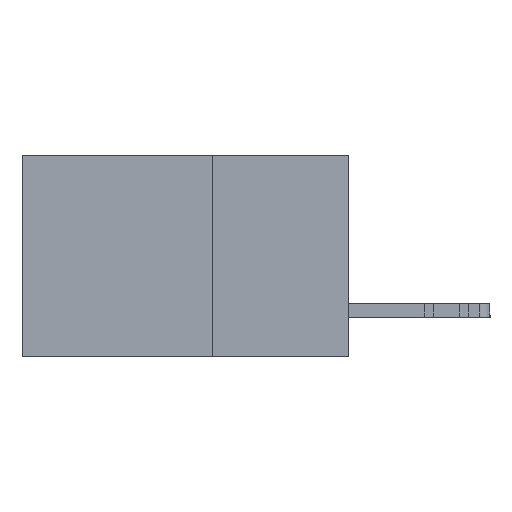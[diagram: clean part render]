
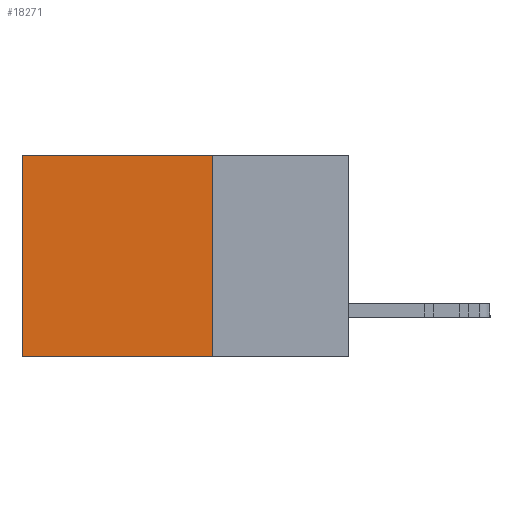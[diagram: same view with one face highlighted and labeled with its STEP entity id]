
A CAD part, left-side view. The second image highlights one B-rep face of the part: STEP entity #18271.
In plain terms, the highlighted planar face has unit normal (-1, 0, 0).
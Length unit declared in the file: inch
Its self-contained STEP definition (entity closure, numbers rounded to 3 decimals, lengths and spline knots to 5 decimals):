
#656 = LINE ( 'NONE', #15399, #14418 ) ;
#1472 = CARTESIAN_POINT ( 'NONE',  ( 0.298, 0.6, 0. ) ) ;
#2186 = EDGE_CURVE ( 'NONE', #17357, #15263, #656, .T. ) ;
#2240 = CARTESIAN_POINT ( 'NONE',  ( 0.298, 0.6, -0.37 ) ) ;
#2819 = DIRECTION ( 'NONE',  ( 1., 0., 0. ) ) ;
#4165 = DIRECTION ( 'NONE',  ( 0., 1., 0. ) ) ;
#5408 = PLANE ( 'NONE',  #13790 ) ;
#6803 = CARTESIAN_POINT ( 'NONE',  ( 0.298, 0.25, -0.37 ) ) ;
#9617 = CARTESIAN_POINT ( 'NONE',  ( 0.298, 0.25, 0. ) ) ;
#9761 = DIRECTION ( 'NONE',  ( 0., 1., 0. ) ) ;
#10037 = LINE ( 'NONE', #1472, #17065 ) ;
#10196 = VERTEX_POINT ( 'NONE', #2240 ) ;
#12437 = CARTESIAN_POINT ( 'NONE',  ( 0.298, 0.6, 0. ) ) ;
#13053 = VERTEX_POINT ( 'NONE', #6803 ) ;
#13790 = AXIS2_PLACEMENT_3D ( 'NONE', #18879, #2819, #28018 ) ;
#14145 = ORIENTED_EDGE ( 'NONE', *, *, #22791, .T. ) ;
#14226 = LINE ( 'NONE', #23444, #23072 ) ;
#14418 = VECTOR ( 'NONE', #4165, 39.37008 ) ;
#15263 = VERTEX_POINT ( 'NONE', #12437 ) ;
#15399 = CARTESIAN_POINT ( 'NONE',  ( 0.298, 0.25, 0. ) ) ;
#15647 = FACE_OUTER_BOUND ( 'NONE', #26648, .T. ) ;
#17065 = VECTOR ( 'NONE', #19205, 39.37008 ) ;
#17357 = VERTEX_POINT ( 'NONE', #9617 ) ;
#17630 = DIRECTION ( 'NONE',  ( 0., 0., -1. ) ) ;
#18271 = ADVANCED_FACE ( 'NONE', ( #15647 ), #5408, .F. ) ;
#18315 = EDGE_CURVE ( 'NONE', #13053, #10196, #14226, .T. ) ;
#18879 = CARTESIAN_POINT ( 'NONE',  ( 0.298, 0.25, 0. ) ) ;
#19205 = DIRECTION ( 'NONE',  ( 0., 0., -1. ) ) ;
#19442 = LINE ( 'NONE', #26662, #22303 ) ;
#22303 = VECTOR ( 'NONE', #17630, 39.37008 ) ;
#22791 = EDGE_CURVE ( 'NONE', #15263, #10196, #10037, .T. ) ;
#23072 = VECTOR ( 'NONE', #9761, 39.37008 ) ;
#23226 = ORIENTED_EDGE ( 'NONE', *, *, #18315, .F. ) ;
#23444 = CARTESIAN_POINT ( 'NONE',  ( 0.298, 0.25, -0.37 ) ) ;
#24437 = EDGE_CURVE ( 'NONE', #17357, #13053, #19442, .T. ) ;
#26648 = EDGE_LOOP ( 'NONE', ( #14145, #23226, #27962, #26735 ) ) ;
#26662 = CARTESIAN_POINT ( 'NONE',  ( 0.298, 0.25, 0. ) ) ;
#26735 = ORIENTED_EDGE ( 'NONE', *, *, #2186, .T. ) ;
#27962 = ORIENTED_EDGE ( 'NONE', *, *, #24437, .F. ) ;
#28018 = DIRECTION ( 'NONE',  ( 0., 0., -1. ) ) ;
